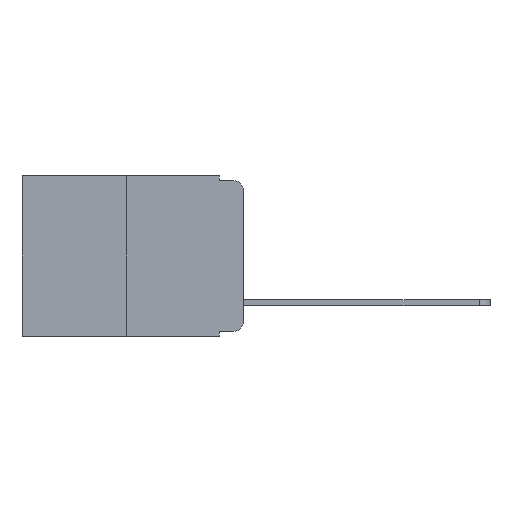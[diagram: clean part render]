
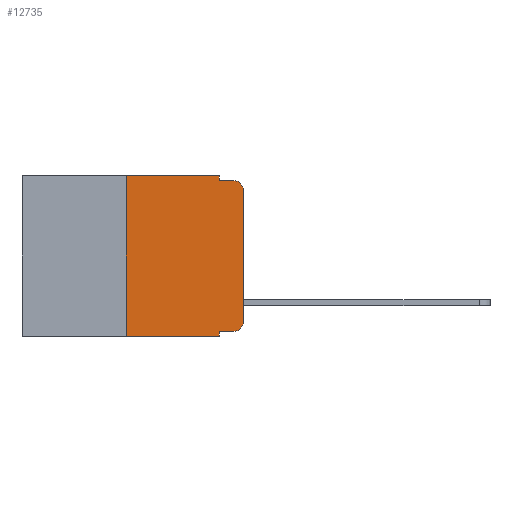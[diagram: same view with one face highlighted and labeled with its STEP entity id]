
A CAD part, left-side view. The second image highlights one B-rep face of the part: STEP entity #12735.
In plain terms, the highlighted planar face has unit normal (-1, 0, 0).
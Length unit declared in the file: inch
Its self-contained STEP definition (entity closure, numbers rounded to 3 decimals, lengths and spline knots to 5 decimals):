
#173 = EDGE_CURVE ( 'NONE', #2125, #3605, #14604, .T. ) ;
#349 = VERTEX_POINT ( 'NONE', #2824 ) ;
#1190 = EDGE_CURVE ( 'NONE', #4658, #349, #6818, .T. ) ;
#1197 = ORIENTED_EDGE ( 'NONE', *, *, #5049, .T. ) ;
#1539 = VECTOR ( 'NONE', #15678, 39.37008 ) ;
#1585 = VERTEX_POINT ( 'NONE', #6578 ) ;
#1604 = CARTESIAN_POINT ( 'NONE',  ( 0., 0.051, 0. ) ) ;
#1642 = ORIENTED_EDGE ( 'NONE', *, *, #2150, .F. ) ;
#1694 = LINE ( 'NONE', #6058, #2603 ) ;
#1966 = VERTEX_POINT ( 'NONE', #16456 ) ;
#1988 = LINE ( 'NONE', #5164, #1539 ) ;
#2058 = LINE ( 'NONE', #9629, #5439 ) ;
#2125 = VERTEX_POINT ( 'NONE', #6520 ) ;
#2130 = CARTESIAN_POINT ( 'NONE',  ( 0., 0.051, 0. ) ) ;
#2147 = VERTEX_POINT ( 'NONE', #14661 ) ;
#2150 = EDGE_CURVE ( 'NONE', #349, #1585, #16749, .T. ) ;
#2381 = VECTOR ( 'NONE', #5665, 39.37008 ) ;
#2592 = VERTEX_POINT ( 'NONE', #4675 ) ;
#2603 = VECTOR ( 'NONE', #7467, 39.37008 ) ;
#2824 = CARTESIAN_POINT ( 'NONE',  ( 0., 0.051, -0.01 ) ) ;
#3071 = VECTOR ( 'NONE', #13361, 39.37008 ) ;
#3115 = EDGE_CURVE ( 'NONE', #11877, #1585, #6752, .T. ) ;
#3122 = DIRECTION ( 'NONE',  ( 0., 0., -1. ) ) ;
#3605 = VERTEX_POINT ( 'NONE', #5719 ) ;
#3747 = DIRECTION ( 'NONE',  ( 0., 0., -1. ) ) ;
#4658 = VERTEX_POINT ( 'NONE', #5999 ) ;
#4675 = CARTESIAN_POINT ( 'NONE',  ( 0., 0.051, -0.343 ) ) ;
#5025 = ORIENTED_EDGE ( 'NONE', *, *, #3115, .T. ) ;
#5049 = EDGE_CURVE ( 'NONE', #1966, #11877, #16586, .T. ) ;
#5073 = CARTESIAN_POINT ( 'NONE',  ( 0., 0.02, -0.03 ) ) ;
#5127 = CARTESIAN_POINT ( 'NONE',  ( 0., 0.473, 0. ) ) ;
#5164 = CARTESIAN_POINT ( 'NONE',  ( 0., 0.051, -0.333 ) ) ;
#5209 = DIRECTION ( 'NONE',  ( -1., 0., 0. ) ) ;
#5230 = DIRECTION ( 'NONE',  ( 0., 0., -1. ) ) ;
#5246 = CARTESIAN_POINT ( 'NONE',  ( 0., 0.02, -0.333 ) ) ;
#5315 = EDGE_CURVE ( 'NONE', #3605, #4658, #1694, .T. ) ;
#5439 = VECTOR ( 'NONE', #7030, 39.37008 ) ;
#5665 = DIRECTION ( 'NONE',  ( 0., 0., 1. ) ) ;
#5719 = CARTESIAN_POINT ( 'NONE',  ( 0., 0.25, 0. ) ) ;
#5999 = CARTESIAN_POINT ( 'NONE',  ( 0., 0.051, 0. ) ) ;
#6058 = CARTESIAN_POINT ( 'NONE',  ( 0., 0.473, 0. ) ) ;
#6511 = DIRECTION ( 'NONE',  ( -1., 0., 0. ) ) ;
#6520 = CARTESIAN_POINT ( 'NONE',  ( 0., 0.25, -0.343 ) ) ;
#6578 = CARTESIAN_POINT ( 'NONE',  ( 0., 0.02, -0.01 ) ) ;
#6752 = CIRCLE ( 'NONE', #11488, 0.02 ) ;
#6818 = LINE ( 'NONE', #2130, #3071 ) ;
#7030 = DIRECTION ( 'NONE',  ( 0., -1., 0. ) ) ;
#7142 = EDGE_CURVE ( 'NONE', #2125, #2592, #2058, .T. ) ;
#7467 = DIRECTION ( 'NONE',  ( 0., -1., 0. ) ) ;
#7860 = CARTESIAN_POINT ( 'NONE',  ( 0., 0.25, 0. ) ) ;
#8420 = CIRCLE ( 'NONE', #11060, 0.02 ) ;
#8728 = LINE ( 'NONE', #1604, #15228 ) ;
#9177 = PLANE ( 'NONE',  #13233 ) ;
#9418 = ORIENTED_EDGE ( 'NONE', *, *, #1190, .F. ) ;
#9629 = CARTESIAN_POINT ( 'NONE',  ( 0., 0.473, -0.343 ) ) ;
#9806 = ORIENTED_EDGE ( 'NONE', *, *, #7142, .T. ) ;
#11060 = AXIS2_PLACEMENT_3D ( 'NONE', #14313, #6511, #15639 ) ;
#11075 = DIRECTION ( 'NONE',  ( 0., 0., 1. ) ) ;
#11488 = AXIS2_PLACEMENT_3D ( 'NONE', #5073, #5209, #5230 ) ;
#11577 = EDGE_CURVE ( 'NONE', #12775, #1966, #8420, .T. ) ;
#11768 = DIRECTION ( 'NONE',  ( 1., 0., 0. ) ) ;
#11877 = VERTEX_POINT ( 'NONE', #16511 ) ;
#12735 = ADVANCED_FACE ( 'NONE', ( #15662 ), #9177, .F. ) ;
#12775 = VERTEX_POINT ( 'NONE', #5246 ) ;
#12849 = ORIENTED_EDGE ( 'NONE', *, *, #5315, .F. ) ;
#13233 = AXIS2_PLACEMENT_3D ( 'NONE', #5127, #11768, #3747 ) ;
#13267 = ORIENTED_EDGE ( 'NONE', *, *, #14191, .F. ) ;
#13303 = VECTOR ( 'NONE', #16901, 39.37008 ) ;
#13325 = EDGE_CURVE ( 'NONE', #2147, #12775, #1988, .T. ) ;
#13361 = DIRECTION ( 'NONE',  ( 0., 0., -1. ) ) ;
#13478 = CARTESIAN_POINT ( 'NONE',  ( 0., 0.051, -0.01 ) ) ;
#13677 = ORIENTED_EDGE ( 'NONE', *, *, #13325, .T. ) ;
#13958 = CARTESIAN_POINT ( 'NONE',  ( 0., 0., 0. ) ) ;
#14177 = VECTOR ( 'NONE', #11075, 39.37008 ) ;
#14191 = EDGE_CURVE ( 'NONE', #2147, #2592, #8728, .T. ) ;
#14313 = CARTESIAN_POINT ( 'NONE',  ( 0., 0.02, -0.313 ) ) ;
#14604 = LINE ( 'NONE', #7860, #14177 ) ;
#14661 = CARTESIAN_POINT ( 'NONE',  ( 0., 0.051, -0.333 ) ) ;
#15228 = VECTOR ( 'NONE', #3122, 39.37008 ) ;
#15266 = EDGE_LOOP ( 'NONE', ( #1197, #5025, #1642, #9418, #12849, #16327, #9806, #13267, #13677, #16884 ) ) ;
#15639 = DIRECTION ( 'NONE',  ( 0., 0., -1. ) ) ;
#15662 = FACE_OUTER_BOUND ( 'NONE', #15266, .T. ) ;
#15678 = DIRECTION ( 'NONE',  ( 0., -1., 0. ) ) ;
#16327 = ORIENTED_EDGE ( 'NONE', *, *, #173, .F. ) ;
#16456 = CARTESIAN_POINT ( 'NONE',  ( 0., 0., -0.313 ) ) ;
#16511 = CARTESIAN_POINT ( 'NONE',  ( 0., 0., -0.03 ) ) ;
#16586 = LINE ( 'NONE', #13958, #2381 ) ;
#16749 = LINE ( 'NONE', #13478, #13303 ) ;
#16884 = ORIENTED_EDGE ( 'NONE', *, *, #11577, .T. ) ;
#16901 = DIRECTION ( 'NONE',  ( 0., -1., 0. ) ) ;
